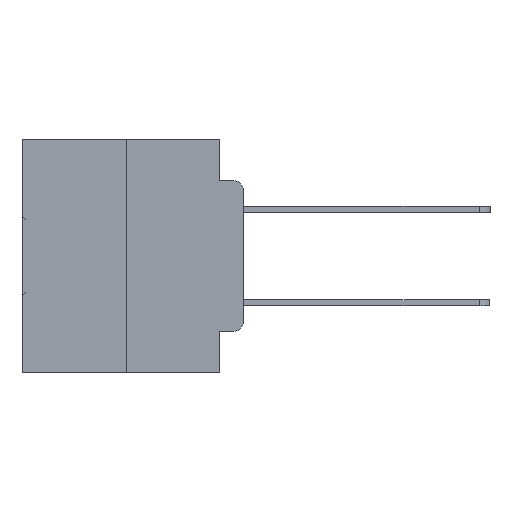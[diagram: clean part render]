
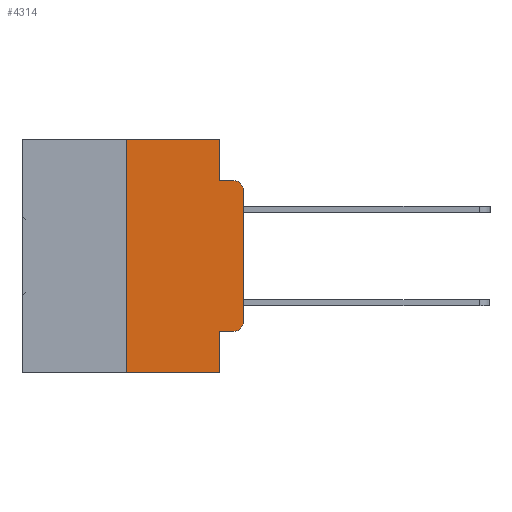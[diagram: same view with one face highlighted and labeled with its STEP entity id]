
A CAD part, left-side view. The second image highlights one B-rep face of the part: STEP entity #4314.
In plain terms, the highlighted planar face has unit normal (-1, 0, 0).
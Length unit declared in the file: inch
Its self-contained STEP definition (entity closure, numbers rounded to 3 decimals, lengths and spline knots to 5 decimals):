
#110 = CARTESIAN_POINT ( 'NONE',  ( 0., 0.02, -0.3915 ) ) ;
#210 = VERTEX_POINT ( 'NONE', #24094 ) ;
#1001 = ORIENTED_EDGE ( 'NONE', *, *, #35761, .F. ) ;
#1346 = VECTOR ( 'NONE', #21009, 39.37008 ) ;
#1372 = CARTESIAN_POINT ( 'NONE',  ( 0., 0.02, -0.0885 ) ) ;
#1445 = ORIENTED_EDGE ( 'NONE', *, *, #15976, .F. ) ;
#1833 = VECTOR ( 'NONE', #31487, 39.37008 ) ;
#2900 = DIRECTION ( 'NONE',  ( 0., 0., -1. ) ) ;
#2904 = EDGE_CURVE ( 'NONE', #210, #20653, #14758, .T. ) ;
#3554 = LINE ( 'NONE', #23801, #17553 ) ;
#3846 = CARTESIAN_POINT ( 'NONE',  ( 0., 0., 0. ) ) ;
#4314 = ADVANCED_FACE ( 'NONE', ( #11127 ), #13880, .F. ) ;
#5874 = VERTEX_POINT ( 'NONE', #7241 ) ;
#7241 = CARTESIAN_POINT ( 'NONE',  ( 0., 0.051, 0. ) ) ;
#7520 = EDGE_CURVE ( 'NONE', #5874, #9389, #29622, .T. ) ;
#7568 = EDGE_CURVE ( 'NONE', #14209, #31738, #22274, .T. ) ;
#7627 = VECTOR ( 'NONE', #13253, 39.37008 ) ;
#8704 = LINE ( 'NONE', #31960, #1346 ) ;
#8816 = ORIENTED_EDGE ( 'NONE', *, *, #30540, .F. ) ;
#9266 = ORIENTED_EDGE ( 'NONE', *, *, #7520, .F. ) ;
#9389 = VERTEX_POINT ( 'NONE', #28720 ) ;
#10108 = ORIENTED_EDGE ( 'NONE', *, *, #16035, .T. ) ;
#10384 = LINE ( 'NONE', #35636, #25138 ) ;
#11127 = FACE_OUTER_BOUND ( 'NONE', #24494, .T. ) ;
#12181 = CARTESIAN_POINT ( 'NONE',  ( 0., 0.051, 0. ) ) ;
#12207 = DIRECTION ( 'NONE',  ( 0., 0., 1. ) ) ;
#13253 = DIRECTION ( 'NONE',  ( 0., 0., 1. ) ) ;
#13400 = VERTEX_POINT ( 'NONE', #20952 ) ;
#13880 = PLANE ( 'NONE',  #16259 ) ;
#14087 = CARTESIAN_POINT ( 'NONE',  ( 0., 0., -0.3915 ) ) ;
#14209 = VERTEX_POINT ( 'NONE', #21252 ) ;
#14284 = VERTEX_POINT ( 'NONE', #16210 ) ;
#14758 = CIRCLE ( 'NONE', #15986, 0.02 ) ;
#15124 = LINE ( 'NONE', #24249, #7627 ) ;
#15774 = EDGE_CURVE ( 'NONE', #32916, #17120, #21970, .T. ) ;
#15976 = EDGE_CURVE ( 'NONE', #13400, #5874, #29734, .T. ) ;
#15986 = AXIS2_PLACEMENT_3D ( 'NONE', #21787, #29667, #29625 ) ;
#16035 = EDGE_CURVE ( 'NONE', #17120, #210, #34401, .T. ) ;
#16210 = CARTESIAN_POINT ( 'NONE',  ( 0., 0.051, -0.4115 ) ) ;
#16259 = AXIS2_PLACEMENT_3D ( 'NONE', #24866, #33142, #16691 ) ;
#16286 = ORIENTED_EDGE ( 'NONE', *, *, #2904, .T. ) ;
#16691 = DIRECTION ( 'NONE',  ( 0., 0., -1. ) ) ;
#16768 = ORIENTED_EDGE ( 'NONE', *, *, #15774, .T. ) ;
#17120 = VERTEX_POINT ( 'NONE', #14087 ) ;
#17553 = VECTOR ( 'NONE', #29353, 39.37008 ) ;
#19215 = DIRECTION ( 'NONE',  ( 0., -1., 0. ) ) ;
#19447 = EDGE_CURVE ( 'NONE', #14284, #32916, #3554, .T. ) ;
#19586 = DIRECTION ( 'NONE',  ( -1., 0., 0. ) ) ;
#20306 = DIRECTION ( 'NONE',  ( 0., -1., 0. ) ) ;
#20545 = VECTOR ( 'NONE', #26166, 39.37008 ) ;
#20606 = ORIENTED_EDGE ( 'NONE', *, *, #7568, .T. ) ;
#20653 = VERTEX_POINT ( 'NONE', #1372 ) ;
#20952 = CARTESIAN_POINT ( 'NONE',  ( 0., 0.25, 0. ) ) ;
#21009 = DIRECTION ( 'NONE',  ( 0., 0., -1. ) ) ;
#21252 = CARTESIAN_POINT ( 'NONE',  ( 0., 0.25, -0.5 ) ) ;
#21315 = CARTESIAN_POINT ( 'NONE',  ( 0., 0.02, -0.4115 ) ) ;
#21787 = CARTESIAN_POINT ( 'NONE',  ( 0., 0.02, -0.1085 ) ) ;
#21970 = CIRCLE ( 'NONE', #30122, 0.02 ) ;
#22274 = LINE ( 'NONE', #28827, #20545 ) ;
#22335 = ORIENTED_EDGE ( 'NONE', *, *, #28692, .F. ) ;
#23068 = CARTESIAN_POINT ( 'NONE',  ( 0., 0.473, 0. ) ) ;
#23801 = CARTESIAN_POINT ( 'NONE',  ( 0., 0.051, -0.4115 ) ) ;
#24094 = CARTESIAN_POINT ( 'NONE',  ( 0., 0., -0.1085 ) ) ;
#24249 = CARTESIAN_POINT ( 'NONE',  ( 0., 0.25, 0. ) ) ;
#24494 = EDGE_LOOP ( 'NONE', ( #10108, #16286, #1001, #9266, #1445, #8816, #20606, #22335, #29682, #16768 ) ) ;
#24866 = CARTESIAN_POINT ( 'NONE',  ( 0., 0.473, 0. ) ) ;
#25138 = VECTOR ( 'NONE', #19215, 39.37008 ) ;
#26166 = DIRECTION ( 'NONE',  ( 0., -1., 0. ) ) ;
#28692 = EDGE_CURVE ( 'NONE', #14284, #31738, #8704, .T. ) ;
#28720 = CARTESIAN_POINT ( 'NONE',  ( 0., 0.051, -0.0885 ) ) ;
#28827 = CARTESIAN_POINT ( 'NONE',  ( 0., 0.473, -0.5 ) ) ;
#28862 = VECTOR ( 'NONE', #20306, 39.37008 ) ;
#29353 = DIRECTION ( 'NONE',  ( 0., -1., 0. ) ) ;
#29622 = LINE ( 'NONE', #12181, #1833 ) ;
#29625 = DIRECTION ( 'NONE',  ( 0., 0., -1. ) ) ;
#29667 = DIRECTION ( 'NONE',  ( -1., 0., 0. ) ) ;
#29682 = ORIENTED_EDGE ( 'NONE', *, *, #19447, .T. ) ;
#29734 = LINE ( 'NONE', #23068, #28862 ) ;
#30122 = AXIS2_PLACEMENT_3D ( 'NONE', #110, #19586, #2900 ) ;
#30540 = EDGE_CURVE ( 'NONE', #14209, #13400, #15124, .T. ) ;
#31487 = DIRECTION ( 'NONE',  ( 0., 0., -1. ) ) ;
#31738 = VERTEX_POINT ( 'NONE', #32331 ) ;
#31960 = CARTESIAN_POINT ( 'NONE',  ( 0., 0.051, 0. ) ) ;
#32331 = CARTESIAN_POINT ( 'NONE',  ( 0., 0.051, -0.5 ) ) ;
#32916 = VERTEX_POINT ( 'NONE', #21315 ) ;
#33142 = DIRECTION ( 'NONE',  ( 1., 0., 0. ) ) ;
#33580 = VECTOR ( 'NONE', #12207, 39.37008 ) ;
#34401 = LINE ( 'NONE', #3846, #33580 ) ;
#35636 = CARTESIAN_POINT ( 'NONE',  ( 0., 0.051, -0.0885 ) ) ;
#35761 = EDGE_CURVE ( 'NONE', #9389, #20653, #10384, .T. ) ;
